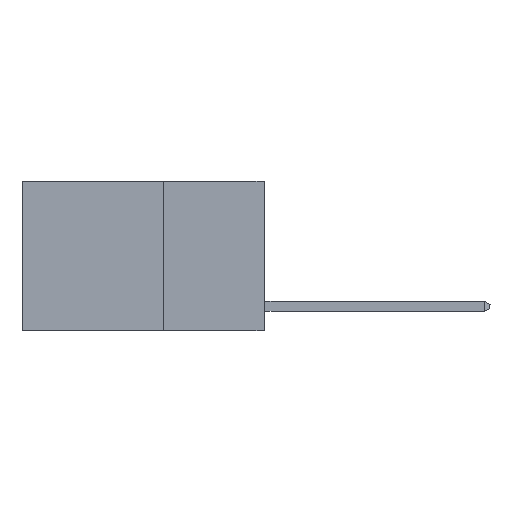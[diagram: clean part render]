
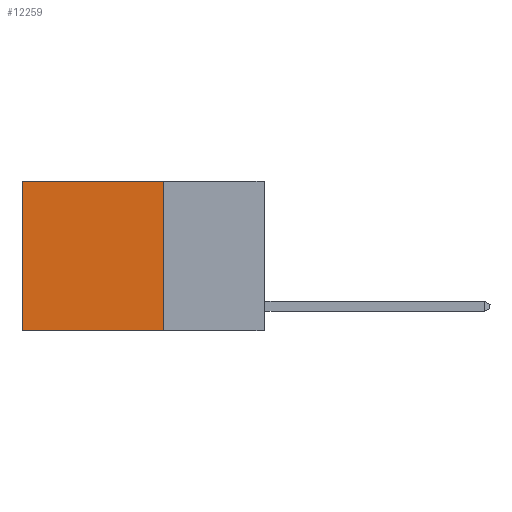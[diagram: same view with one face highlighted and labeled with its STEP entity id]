
A CAD part, left-side view. The second image highlights one B-rep face of the part: STEP entity #12259.
In plain terms, the highlighted planar face has unit normal (-1, 0, 0).
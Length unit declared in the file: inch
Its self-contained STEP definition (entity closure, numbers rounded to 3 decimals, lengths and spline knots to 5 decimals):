
#482 = VECTOR ( 'NONE', #10597, 39.37008 ) ;
#750 = VERTEX_POINT ( 'NONE', #18259 ) ;
#1104 = EDGE_LOOP ( 'NONE', ( #12511, #3534, #3597, #14612 ) ) ;
#2197 = CARTESIAN_POINT ( 'NONE',  ( 0.2625, 0.6, 0. ) ) ;
#3208 = CARTESIAN_POINT ( 'NONE',  ( 0.2625, 0.6, 0. ) ) ;
#3532 = EDGE_CURVE ( 'NONE', #750, #12330, #13861, .T. ) ;
#3534 = ORIENTED_EDGE ( 'NONE', *, *, #3532, .F. ) ;
#3597 = ORIENTED_EDGE ( 'NONE', *, *, #19160, .F. ) ;
#3906 = CARTESIAN_POINT ( 'NONE',  ( 0.2625, 0.25, 0. ) ) ;
#4960 = FACE_OUTER_BOUND ( 'NONE', #1104, .T. ) ;
#5677 = LINE ( 'NONE', #8740, #17335 ) ;
#5712 = PLANE ( 'NONE',  #14004 ) ;
#6030 = CARTESIAN_POINT ( 'NONE',  ( 0.2625, 0.25, 0. ) ) ;
#6254 = EDGE_CURVE ( 'NONE', #17774, #12330, #12099, .T. ) ;
#6350 = DIRECTION ( 'NONE',  ( 0., 0., -1. ) ) ;
#7259 = DIRECTION ( 'NONE',  ( 1., 0., 0. ) ) ;
#7575 = DIRECTION ( 'NONE',  ( 0., 1., 0. ) ) ;
#7858 = VERTEX_POINT ( 'NONE', #3906 ) ;
#8010 = VECTOR ( 'NONE', #6350, 39.37008 ) ;
#8740 = CARTESIAN_POINT ( 'NONE',  ( 0.2625, 0.25, 0. ) ) ;
#9068 = CARTESIAN_POINT ( 'NONE',  ( 0.2625, 0.25, -0.37 ) ) ;
#10597 = DIRECTION ( 'NONE',  ( 0., 1., 0. ) ) ;
#11839 = CARTESIAN_POINT ( 'NONE',  ( 0.2625, 0.25, 0. ) ) ;
#12099 = LINE ( 'NONE', #3208, #8010 ) ;
#12259 = ADVANCED_FACE ( 'NONE', ( #4960 ), #5712, .F. ) ;
#12330 = VERTEX_POINT ( 'NONE', #18028 ) ;
#12511 = ORIENTED_EDGE ( 'NONE', *, *, #6254, .T. ) ;
#13861 = LINE ( 'NONE', #9068, #482 ) ;
#14004 = AXIS2_PLACEMENT_3D ( 'NONE', #11839, #7259, #17833 ) ;
#14612 = ORIENTED_EDGE ( 'NONE', *, *, #15985, .T. ) ;
#15985 = EDGE_CURVE ( 'NONE', #7858, #17774, #17484, .T. ) ;
#17037 = VECTOR ( 'NONE', #7575, 39.37008 ) ;
#17335 = VECTOR ( 'NONE', #17655, 39.37008 ) ;
#17484 = LINE ( 'NONE', #6030, #17037 ) ;
#17655 = DIRECTION ( 'NONE',  ( 0., 0., -1. ) ) ;
#17774 = VERTEX_POINT ( 'NONE', #2197 ) ;
#17833 = DIRECTION ( 'NONE',  ( 0., 0., -1. ) ) ;
#18028 = CARTESIAN_POINT ( 'NONE',  ( 0.2625, 0.6, -0.37 ) ) ;
#18259 = CARTESIAN_POINT ( 'NONE',  ( 0.2625, 0.25, -0.37 ) ) ;
#19160 = EDGE_CURVE ( 'NONE', #7858, #750, #5677, .T. ) ;
